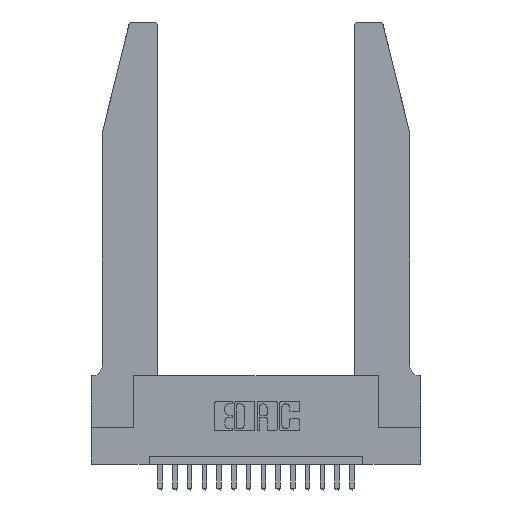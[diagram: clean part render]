
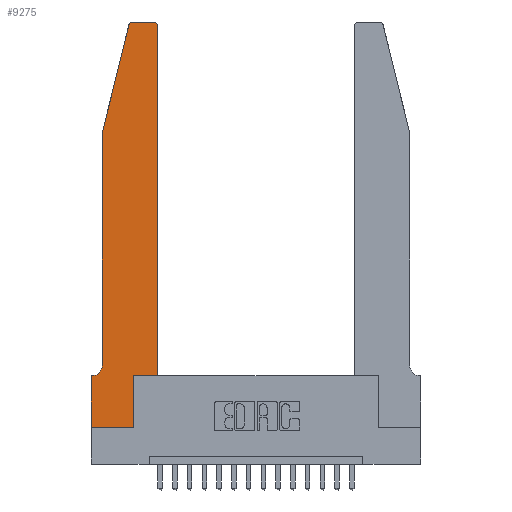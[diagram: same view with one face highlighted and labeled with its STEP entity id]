
A CAD part, top view. The second image highlights one B-rep face of the part: STEP entity #9275.
In plain terms, the highlighted planar face has unit normal (0, 0, 1).
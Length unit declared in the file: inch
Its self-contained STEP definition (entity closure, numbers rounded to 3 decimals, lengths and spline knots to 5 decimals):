
#101 = VECTOR ( 'NONE', #5947, 39.37008 ) ;
#255 = EDGE_CURVE ( 'NONE', #7786, #8357, #499, .T. ) ;
#385 = CARTESIAN_POINT ( 'NONE',  ( 0.4205, 2.72, 0.37 ) ) ;
#498 = DIRECTION ( 'NONE',  ( 1., 0., 0. ) ) ;
#499 = LINE ( 'NONE', #12012, #14822 ) ;
#1878 = VERTEX_POINT ( 'NONE', #14617 ) ;
#1922 = DIRECTION ( 'NONE',  ( 0., 0., 1. ) ) ;
#1967 = DIRECTION ( 'NONE',  ( 0., -1., 0. ) ) ;
#2352 = VERTEX_POINT ( 'NONE', #9700 ) ;
#2489 = LINE ( 'NONE', #15568, #8763 ) ;
#2588 = CIRCLE ( 'NONE', #7916, 0.03 ) ;
#2660 = CARTESIAN_POINT ( 'NONE',  ( 0.4505, 0.35, 0.37 ) ) ;
#2878 = DIRECTION ( 'NONE',  ( 1., 0., 0. ) ) ;
#2935 = VECTOR ( 'NONE', #17065, 39.37008 ) ;
#3061 = DIRECTION ( 'NONE',  ( 0., 1., 0. ) ) ;
#3696 = EDGE_CURVE ( 'NONE', #13062, #11829, #9837, .T. ) ;
#3799 = CARTESIAN_POINT ( 'NONE',  ( 0.25487, 2.72718, 0.37 ) ) ;
#4008 = LINE ( 'NONE', #17845, #101 ) ;
#4081 = CARTESIAN_POINT ( 'NONE',  ( 0.2865, 0.35, 0.37 ) ) ;
#4912 = CARTESIAN_POINT ( 'NONE',  ( 0.2865, 0., 0.37 ) ) ;
#4959 = AXIS2_PLACEMENT_3D ( 'NONE', #13236, #8987, #10482 ) ;
#5257 = CARTESIAN_POINT ( 'NONE',  ( 0.4505, 0.35, 0.37 ) ) ;
#5359 = ORIENTED_EDGE ( 'NONE', *, *, #5874, .T. ) ;
#5716 = AXIS2_PLACEMENT_3D ( 'NONE', #10093, #7142, #14698 ) ;
#5874 = EDGE_CURVE ( 'NONE', #8878, #10939, #2588, .T. ) ;
#5947 = DIRECTION ( 'NONE',  ( -1., 0., 0. ) ) ;
#6164 = VECTOR ( 'NONE', #1967, 39.37008 ) ;
#6228 = EDGE_CURVE ( 'NONE', #11412, #13062, #12959, .T. ) ;
#6399 = ORIENTED_EDGE ( 'NONE', *, *, #19173, .T. ) ;
#6470 = CARTESIAN_POINT ( 'NONE',  ( 0.0755, 0.42, 0.37 ) ) ;
#7078 = CARTESIAN_POINT ( 'NONE',  ( 0.4505, 0.35, 0.37 ) ) ;
#7142 = DIRECTION ( 'NONE',  ( 0., 0., -1. ) ) ;
#7206 = VECTOR ( 'NONE', #3061, 39.37008 ) ;
#7296 = ORIENTED_EDGE ( 'NONE', *, *, #10554, .T. ) ;
#7502 = DIRECTION ( 'NONE',  ( 0., -1., 0. ) ) ;
#7556 = ORIENTED_EDGE ( 'NONE', *, *, #15191, .T. ) ;
#7786 = VERTEX_POINT ( 'NONE', #17375 ) ;
#7916 = AXIS2_PLACEMENT_3D ( 'NONE', #8983, #12783, #9646 ) ;
#8336 = DIRECTION ( 'NONE',  ( -1., 0., 0. ) ) ;
#8357 = VERTEX_POINT ( 'NONE', #15943 ) ;
#8445 = EDGE_CURVE ( 'NONE', #11829, #2352, #11748, .T. ) ;
#8464 = CARTESIAN_POINT ( 'NONE',  ( 0.2605, 2.75, 0.37 ) ) ;
#8763 = VECTOR ( 'NONE', #15497, 39.37008 ) ;
#8878 = VERTEX_POINT ( 'NONE', #17770 ) ;
#8983 = CARTESIAN_POINT ( 'NONE',  ( 0.284, 2.72, 0.37 ) ) ;
#8987 = DIRECTION ( 'NONE',  ( 0., 0., 1. ) ) ;
#9197 = VECTOR ( 'NONE', #8336, 39.37008 ) ;
#9275 = ADVANCED_FACE ( 'NONE', ( #10933 ), #17833, .T. ) ;
#9619 = EDGE_CURVE ( 'NONE', #14897, #17647, #16654, .T. ) ;
#9646 = DIRECTION ( 'NONE',  ( 1., 0., 0. ) ) ;
#9700 = CARTESIAN_POINT ( 'NONE',  ( 0.4505, 2.72, 0.37 ) ) ;
#9837 = LINE ( 'NONE', #7078, #10070 ) ;
#9886 = LINE ( 'NONE', #13847, #6164 ) ;
#10070 = VECTOR ( 'NONE', #2878, 39.37008 ) ;
#10093 = CARTESIAN_POINT ( 'NONE',  ( 0.0055, 0.42, 0.37 ) ) ;
#10482 = DIRECTION ( 'NONE',  ( 1., 0., 0. ) ) ;
#10554 = EDGE_CURVE ( 'NONE', #10939, #12912, #12458, .T. ) ;
#10655 = ORIENTED_EDGE ( 'NONE', *, *, #6228, .T. ) ;
#10933 = FACE_OUTER_BOUND ( 'NONE', #15944, .T. ) ;
#10939 = VERTEX_POINT ( 'NONE', #3799 ) ;
#11412 = VERTEX_POINT ( 'NONE', #4912 ) ;
#11748 = LINE ( 'NONE', #5257, #2935 ) ;
#11829 = VERTEX_POINT ( 'NONE', #2660 ) ;
#12012 = CARTESIAN_POINT ( 'NONE',  ( 0., 0., 0.37 ) ) ;
#12458 = LINE ( 'NONE', #14173, #14318 ) ;
#12614 = CARTESIAN_POINT ( 'NONE',  ( 0.0755, 2., 0.37 ) ) ;
#12783 = DIRECTION ( 'NONE',  ( 0., 0., 1. ) ) ;
#12906 = ORIENTED_EDGE ( 'NONE', *, *, #9619, .T. ) ;
#12912 = VERTEX_POINT ( 'NONE', #12614 ) ;
#12959 = LINE ( 'NONE', #17500, #7206 ) ;
#12987 = EDGE_CURVE ( 'NONE', #1878, #8878, #13102, .T. ) ;
#13014 = AXIS2_PLACEMENT_3D ( 'NONE', #385, #1922, #498 ) ;
#13062 = VERTEX_POINT ( 'NONE', #4081 ) ;
#13102 = LINE ( 'NONE', #8464, #9197 ) ;
#13236 = CARTESIAN_POINT ( 'NONE',  ( 0., 0.35, 0.37 ) ) ;
#13808 = CIRCLE ( 'NONE', #13014, 0.03 ) ;
#13847 = CARTESIAN_POINT ( 'NONE',  ( 0.0755, 2., 0.37 ) ) ;
#14173 = CARTESIAN_POINT ( 'NONE',  ( 0.0755, 2., 0.37 ) ) ;
#14318 = VECTOR ( 'NONE', #17409, 39.37008 ) ;
#14369 = ORIENTED_EDGE ( 'NONE', *, *, #8445, .T. ) ;
#14550 = CARTESIAN_POINT ( 'NONE',  ( 0.0055, 0.35, 0.37 ) ) ;
#14617 = CARTESIAN_POINT ( 'NONE',  ( 0.4205, 2.75, 0.37 ) ) ;
#14698 = DIRECTION ( 'NONE',  ( -1., 0., 0. ) ) ;
#14822 = VECTOR ( 'NONE', #7502, 39.37008 ) ;
#14897 = VERTEX_POINT ( 'NONE', #6470 ) ;
#15191 = EDGE_CURVE ( 'NONE', #17647, #7786, #4008, .T. ) ;
#15304 = ORIENTED_EDGE ( 'NONE', *, *, #17496, .T. ) ;
#15497 = DIRECTION ( 'NONE',  ( 1., 0., 0. ) ) ;
#15512 = ORIENTED_EDGE ( 'NONE', *, *, #12987, .T. ) ;
#15568 = CARTESIAN_POINT ( 'NONE',  ( 0., 0., 0.37 ) ) ;
#15943 = CARTESIAN_POINT ( 'NONE',  ( 0., 0., 0.37 ) ) ;
#15944 = EDGE_LOOP ( 'NONE', ( #15512, #5359, #7296, #6399, #12906, #7556, #19041, #15304, #10655, #16709, #14369, #19117 ) ) ;
#16654 = CIRCLE ( 'NONE', #5716, 0.07 ) ;
#16709 = ORIENTED_EDGE ( 'NONE', *, *, #3696, .T. ) ;
#17065 = DIRECTION ( 'NONE',  ( 0., 1., 0. ) ) ;
#17375 = CARTESIAN_POINT ( 'NONE',  ( 0., 0.35, 0.37 ) ) ;
#17409 = DIRECTION ( 'NONE',  ( -0.239, -0.971, 0. ) ) ;
#17496 = EDGE_CURVE ( 'NONE', #8357, #11412, #2489, .T. ) ;
#17500 = CARTESIAN_POINT ( 'NONE',  ( 0.2865, 0.35, 0.37 ) ) ;
#17647 = VERTEX_POINT ( 'NONE', #14550 ) ;
#17770 = CARTESIAN_POINT ( 'NONE',  ( 0.284, 2.75, 0.37 ) ) ;
#17833 = PLANE ( 'NONE',  #4959 ) ;
#17845 = CARTESIAN_POINT ( 'NONE',  ( 0.0755, 0.35, 0.37 ) ) ;
#18565 = EDGE_CURVE ( 'NONE', #2352, #1878, #13808, .T. ) ;
#19041 = ORIENTED_EDGE ( 'NONE', *, *, #255, .T. ) ;
#19117 = ORIENTED_EDGE ( 'NONE', *, *, #18565, .T. ) ;
#19173 = EDGE_CURVE ( 'NONE', #12912, #14897, #9886, .T. ) ;
